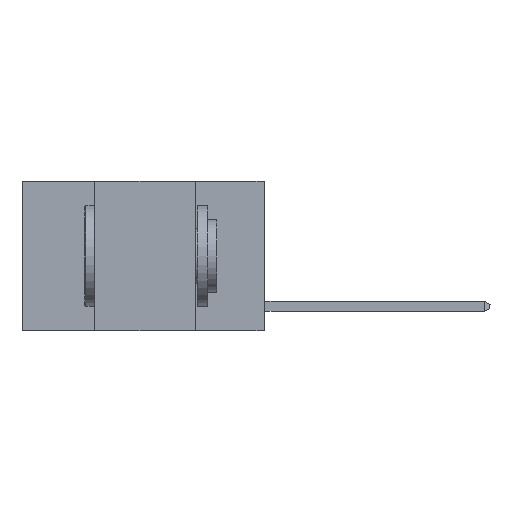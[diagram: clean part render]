
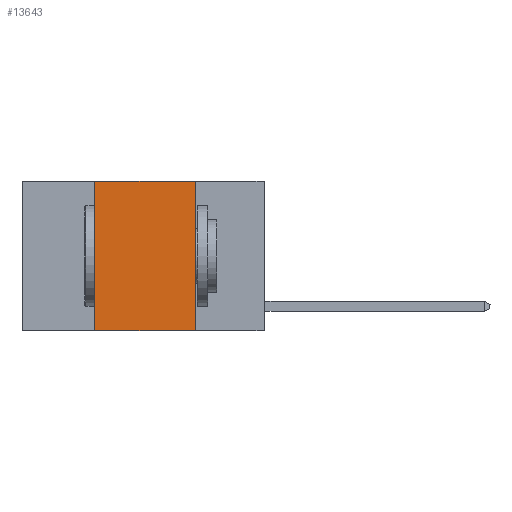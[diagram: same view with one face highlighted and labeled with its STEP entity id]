
A CAD part, left-side view. The second image highlights one B-rep face of the part: STEP entity #13643.
In plain terms, the highlighted planar face has unit normal (-1, 0, 0).
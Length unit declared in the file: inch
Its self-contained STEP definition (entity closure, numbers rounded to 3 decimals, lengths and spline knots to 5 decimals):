
#211 = DIRECTION ( 'NONE',  ( 0., 0., -1. ) ) ;
#810 = ORIENTED_EDGE ( 'NONE', *, *, #16035, .F. ) ;
#1397 = DIRECTION ( 'NONE',  ( 0., 0., 1. ) ) ;
#2437 = AXIS2_PLACEMENT_3D ( 'NONE', #10802, #29037, #6095 ) ;
#3029 = VECTOR ( 'NONE', #5739, 39.37008 ) ;
#4445 = EDGE_CURVE ( 'NONE', #25762, #17831, #5146, .T. ) ;
#5146 = LINE ( 'NONE', #14720, #3029 ) ;
#5299 = FACE_OUTER_BOUND ( 'NONE', #21154, .T. ) ;
#5739 = DIRECTION ( 'NONE',  ( 0., -1., 0. ) ) ;
#6095 = DIRECTION ( 'NONE',  ( 0., 0., -1. ) ) ;
#8956 = VECTOR ( 'NONE', #15818, 39.37008 ) ;
#10344 = VERTEX_POINT ( 'NONE', #15946 ) ;
#10802 = CARTESIAN_POINT ( 'NONE',  ( 0., 0.6, 0. ) ) ;
#11932 = EDGE_CURVE ( 'NONE', #25762, #10344, #28740, .T. ) ;
#12133 = ORIENTED_EDGE ( 'NONE', *, *, #19246, .F. ) ;
#12537 = VERTEX_POINT ( 'NONE', #13746 ) ;
#12699 = ORIENTED_EDGE ( 'NONE', *, *, #11932, .F. ) ;
#13643 = ADVANCED_FACE ( 'NONE', ( #5299 ), #26571, .F. ) ;
#13746 = CARTESIAN_POINT ( 'NONE',  ( 0., 0.17, 0. ) ) ;
#13979 = VECTOR ( 'NONE', #211, 39.37008 ) ;
#14720 = CARTESIAN_POINT ( 'NONE',  ( 0., 0.6, -0.37 ) ) ;
#15253 = VECTOR ( 'NONE', #1397, 39.37008 ) ;
#15275 = LINE ( 'NONE', #29313, #8956 ) ;
#15818 = DIRECTION ( 'NONE',  ( 0., -1., 0. ) ) ;
#15946 = CARTESIAN_POINT ( 'NONE',  ( 0., 0.42, 0. ) ) ;
#16035 = EDGE_CURVE ( 'NONE', #12537, #17831, #26046, .T. ) ;
#17831 = VERTEX_POINT ( 'NONE', #28005 ) ;
#19246 = EDGE_CURVE ( 'NONE', #10344, #12537, #15275, .T. ) ;
#21154 = EDGE_LOOP ( 'NONE', ( #810, #12133, #12699, #22576 ) ) ;
#21907 = CARTESIAN_POINT ( 'NONE',  ( 0., 0.42, -0.37 ) ) ;
#22561 = CARTESIAN_POINT ( 'NONE',  ( 0., 0.17, 0. ) ) ;
#22576 = ORIENTED_EDGE ( 'NONE', *, *, #4445, .T. ) ;
#24258 = CARTESIAN_POINT ( 'NONE',  ( 0., 0.42, 0. ) ) ;
#25762 = VERTEX_POINT ( 'NONE', #21907 ) ;
#26046 = LINE ( 'NONE', #22561, #13979 ) ;
#26571 = PLANE ( 'NONE',  #2437 ) ;
#28005 = CARTESIAN_POINT ( 'NONE',  ( 0., 0.17, -0.37 ) ) ;
#28740 = LINE ( 'NONE', #24258, #15253 ) ;
#29037 = DIRECTION ( 'NONE',  ( 1., 0., 0. ) ) ;
#29313 = CARTESIAN_POINT ( 'NONE',  ( 0., 0.6, 0. ) ) ;
